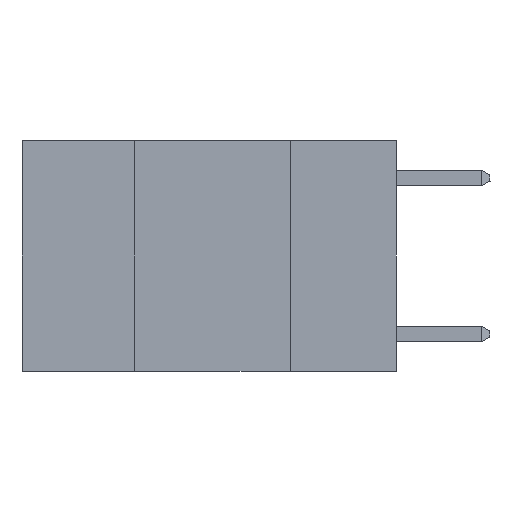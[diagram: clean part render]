
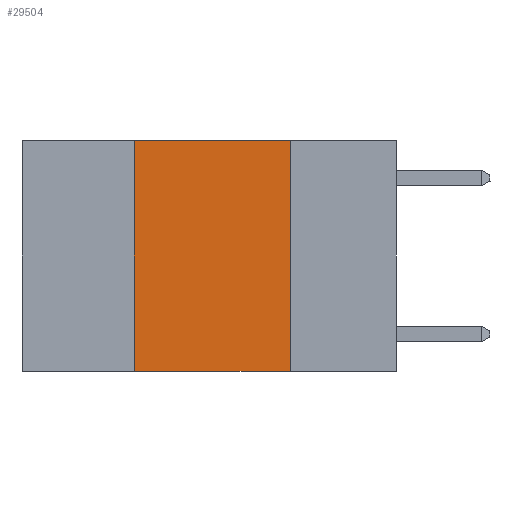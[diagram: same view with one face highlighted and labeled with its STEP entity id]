
A CAD part, left-side view. The second image highlights one B-rep face of the part: STEP entity #29504.
In plain terms, the highlighted planar face has unit normal (-1, 0, 0).
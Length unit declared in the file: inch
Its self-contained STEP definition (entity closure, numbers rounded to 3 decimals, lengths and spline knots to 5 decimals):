
#2211 = VERTEX_POINT ( 'NONE', #19264 ) ;
#3043 = ORIENTED_EDGE ( 'NONE', *, *, #15072, .F. ) ;
#3297 = EDGE_LOOP ( 'NONE', ( #29392, #19389, #3043, #16152 ) ) ;
#3573 = VECTOR ( 'NONE', #25581, 39.37008 ) ;
#3658 = CARTESIAN_POINT ( 'NONE',  ( 0., 0.42, -0.37 ) ) ;
#4222 = VECTOR ( 'NONE', #6376, 39.37008 ) ;
#5031 = VERTEX_POINT ( 'NONE', #15414 ) ;
#5275 = DIRECTION ( 'NONE',  ( 0., 0., 1. ) ) ;
#5483 = CARTESIAN_POINT ( 'NONE',  ( 0., 0.6, 0. ) ) ;
#5877 = DIRECTION ( 'NONE',  ( 0., 0., -1. ) ) ;
#6376 = DIRECTION ( 'NONE',  ( 0., -1., 0. ) ) ;
#7516 = CARTESIAN_POINT ( 'NONE',  ( 0., 0.42, 0. ) ) ;
#9137 = EDGE_CURVE ( 'NONE', #12404, #2211, #28685, .T. ) ;
#10292 = VECTOR ( 'NONE', #5275, 39.37008 ) ;
#10345 = LINE ( 'NONE', #27082, #4222 ) ;
#11031 = LINE ( 'NONE', #7516, #10292 ) ;
#12404 = VERTEX_POINT ( 'NONE', #12982 ) ;
#12982 = CARTESIAN_POINT ( 'NONE',  ( 0., 0.42, 0. ) ) ;
#14008 = AXIS2_PLACEMENT_3D ( 'NONE', #26594, #19882, #5877 ) ;
#15072 = EDGE_CURVE ( 'NONE', #19474, #12404, #11031, .T. ) ;
#15414 = CARTESIAN_POINT ( 'NONE',  ( 0., 0.17, -0.37 ) ) ;
#16152 = ORIENTED_EDGE ( 'NONE', *, *, #22846, .T. ) ;
#17526 = PLANE ( 'NONE',  #14008 ) ;
#19264 = CARTESIAN_POINT ( 'NONE',  ( 0., 0.17, 0. ) ) ;
#19389 = ORIENTED_EDGE ( 'NONE', *, *, #9137, .F. ) ;
#19474 = VERTEX_POINT ( 'NONE', #3658 ) ;
#19783 = EDGE_CURVE ( 'NONE', #2211, #5031, #22122, .T. ) ;
#19882 = DIRECTION ( 'NONE',  ( 1., 0., 0. ) ) ;
#21953 = VECTOR ( 'NONE', #28599, 39.37008 ) ;
#22122 = LINE ( 'NONE', #23303, #3573 ) ;
#22846 = EDGE_CURVE ( 'NONE', #19474, #5031, #10345, .T. ) ;
#23303 = CARTESIAN_POINT ( 'NONE',  ( 0., 0.17, 0. ) ) ;
#25581 = DIRECTION ( 'NONE',  ( 0., 0., -1. ) ) ;
#26594 = CARTESIAN_POINT ( 'NONE',  ( 0., 0.6, 0. ) ) ;
#27082 = CARTESIAN_POINT ( 'NONE',  ( 0., 0.6, -0.37 ) ) ;
#27872 = FACE_OUTER_BOUND ( 'NONE', #3297, .T. ) ;
#28599 = DIRECTION ( 'NONE',  ( 0., -1., 0. ) ) ;
#28685 = LINE ( 'NONE', #5483, #21953 ) ;
#29392 = ORIENTED_EDGE ( 'NONE', *, *, #19783, .F. ) ;
#29504 = ADVANCED_FACE ( 'NONE', ( #27872 ), #17526, .F. ) ;
